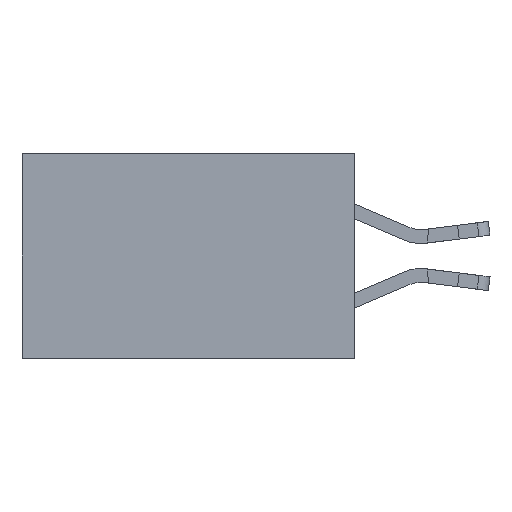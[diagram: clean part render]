
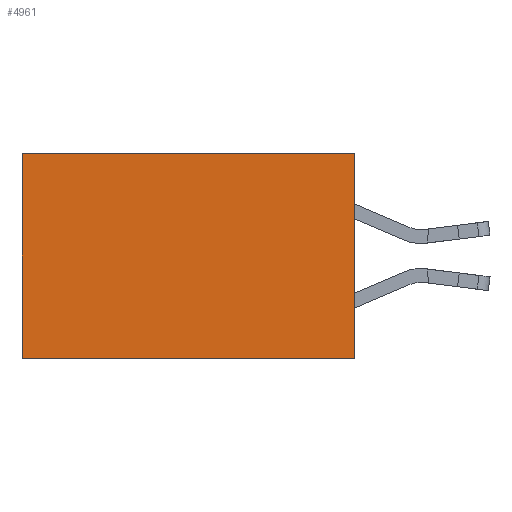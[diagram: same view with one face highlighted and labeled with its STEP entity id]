
A CAD part, left-side view. The second image highlights one B-rep face of the part: STEP entity #4961.
In plain terms, the highlighted planar face has unit normal (-1, 0, 0).
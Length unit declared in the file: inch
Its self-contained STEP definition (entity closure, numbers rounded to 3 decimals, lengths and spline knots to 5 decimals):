
#1060 = VERTEX_POINT ( 'NONE', #14258 ) ;
#1758 = FACE_OUTER_BOUND ( 'NONE', #7479, .T. ) ;
#2681 = DIRECTION ( 'NONE',  ( 0., 0., -1. ) ) ;
#3972 = VECTOR ( 'NONE', #10751, 39.37008 ) ;
#4690 = LINE ( 'NONE', #9904, #10838 ) ;
#4932 = EDGE_CURVE ( 'NONE', #13897, #6580, #10920, .T. ) ;
#4961 = ADVANCED_FACE ( 'NONE', ( #1758 ), #20433, .F. ) ;
#5412 = CARTESIAN_POINT ( 'NONE',  ( 0.298, 0., 0. ) ) ;
#6580 = VERTEX_POINT ( 'NONE', #13749 ) ;
#7479 = EDGE_LOOP ( 'NONE', ( #8990, #11594, #22937, #18616 ) ) ;
#7672 = EDGE_CURVE ( 'NONE', #1060, #6580, #4690, .T. ) ;
#8128 = LINE ( 'NONE', #12079, #3972 ) ;
#8990 = ORIENTED_EDGE ( 'NONE', *, *, #7672, .T. ) ;
#9615 = AXIS2_PLACEMENT_3D ( 'NONE', #13479, #9802, #11578 ) ;
#9632 = VECTOR ( 'NONE', #19788, 39.37008 ) ;
#9802 = DIRECTION ( 'NONE',  ( 1., 0., 0. ) ) ;
#9904 = CARTESIAN_POINT ( 'NONE',  ( 0.298, 0.6, 0. ) ) ;
#10440 = LINE ( 'NONE', #17738, #9632 ) ;
#10598 = CARTESIAN_POINT ( 'NONE',  ( 0.298, 0., -0.37 ) ) ;
#10751 = DIRECTION ( 'NONE',  ( 0., 1., 0. ) ) ;
#10838 = VECTOR ( 'NONE', #2681, 39.37008 ) ;
#10920 = LINE ( 'NONE', #10598, #14785 ) ;
#11578 = DIRECTION ( 'NONE',  ( 0., 0., -1. ) ) ;
#11594 = ORIENTED_EDGE ( 'NONE', *, *, #4932, .F. ) ;
#11901 = EDGE_CURVE ( 'NONE', #12971, #13897, #10440, .T. ) ;
#12079 = CARTESIAN_POINT ( 'NONE',  ( 0.298, 0., 0. ) ) ;
#12971 = VERTEX_POINT ( 'NONE', #5412 ) ;
#13479 = CARTESIAN_POINT ( 'NONE',  ( 0.298, 0., 0. ) ) ;
#13749 = CARTESIAN_POINT ( 'NONE',  ( 0.298, 0.6, -0.37 ) ) ;
#13888 = CARTESIAN_POINT ( 'NONE',  ( 0.298, 0., -0.37 ) ) ;
#13897 = VERTEX_POINT ( 'NONE', #13888 ) ;
#14258 = CARTESIAN_POINT ( 'NONE',  ( 0.298, 0.6, 0. ) ) ;
#14785 = VECTOR ( 'NONE', #15337, 39.37008 ) ;
#15337 = DIRECTION ( 'NONE',  ( 0., 1., 0. ) ) ;
#17738 = CARTESIAN_POINT ( 'NONE',  ( 0.298, 0., 0. ) ) ;
#18108 = EDGE_CURVE ( 'NONE', #12971, #1060, #8128, .T. ) ;
#18616 = ORIENTED_EDGE ( 'NONE', *, *, #18108, .T. ) ;
#19788 = DIRECTION ( 'NONE',  ( 0., 0., -1. ) ) ;
#20433 = PLANE ( 'NONE',  #9615 ) ;
#22937 = ORIENTED_EDGE ( 'NONE', *, *, #11901, .F. ) ;
